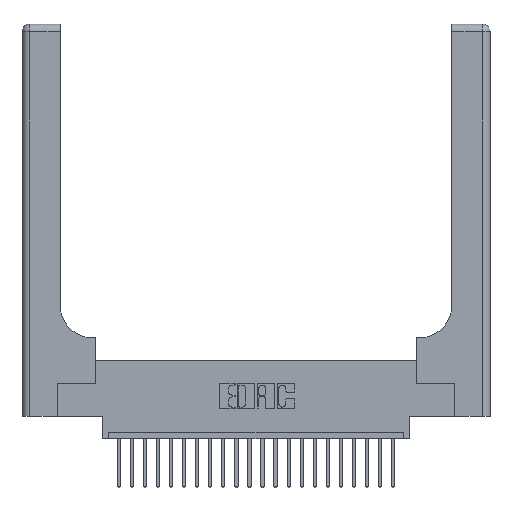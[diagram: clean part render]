
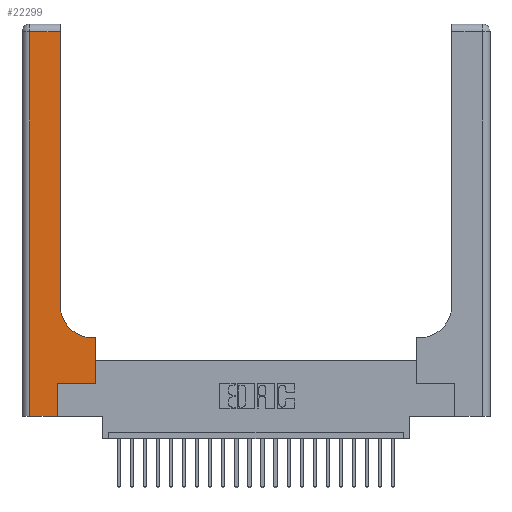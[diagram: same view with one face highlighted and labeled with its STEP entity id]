
A CAD part, top view. The second image highlights one B-rep face of the part: STEP entity #22299.
In plain terms, the highlighted planar face has unit normal (0, 0, 1).
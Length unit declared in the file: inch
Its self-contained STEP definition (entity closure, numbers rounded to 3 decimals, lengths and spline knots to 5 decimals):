
#419 = CARTESIAN_POINT ( 'NONE',  ( 0.269, 0., 0.37 ) ) ;
#493 = DIRECTION ( 'NONE',  ( 0., 0., -1. ) ) ;
#1134 = LINE ( 'NONE', #22113, #18925 ) ;
#1574 = CARTESIAN_POINT ( 'NONE',  ( 0.269, 0.25, 0.37 ) ) ;
#1707 = CARTESIAN_POINT ( 'NONE',  ( 0.06, 0., 0.37 ) ) ;
#3036 = EDGE_CURVE ( 'NONE', #19430, #3932, #19531, .T. ) ;
#3152 = EDGE_CURVE ( 'NONE', #24186, #20681, #1134, .T. ) ;
#3701 = VERTEX_POINT ( 'NONE', #11086 ) ;
#3727 = DIRECTION ( 'NONE',  ( 0., 0., -1. ) ) ;
#3932 = VERTEX_POINT ( 'NONE', #17463 ) ;
#4582 = LINE ( 'NONE', #4952, #14348 ) ;
#4693 = CARTESIAN_POINT ( 'NONE',  ( 0.5585, 0.25, 0.37 ) ) ;
#4952 = CARTESIAN_POINT ( 'NONE',  ( 0., 0., 0.37 ) ) ;
#5368 = DIRECTION ( 'NONE',  ( 1., 0., 0. ) ) ;
#5630 = PLANE ( 'NONE',  #20189 ) ;
#5796 = DIRECTION ( 'NONE',  ( 0., 1., 0. ) ) ;
#7305 = CARTESIAN_POINT ( 'NONE',  ( 0.5585, 0.25, 0.37 ) ) ;
#7680 = EDGE_CURVE ( 'NONE', #3701, #17671, #9521, .T. ) ;
#7905 = ORIENTED_EDGE ( 'NONE', *, *, #16802, .T. ) ;
#7967 = DIRECTION ( 'NONE',  ( 1., 0., 0. ) ) ;
#8793 = FACE_OUTER_BOUND ( 'NONE', #18716, .T. ) ;
#8909 = DIRECTION ( 'NONE',  ( 0., 1., 0. ) ) ;
#9008 = VECTOR ( 'NONE', #12059, 39.37008 ) ;
#9521 = LINE ( 'NONE', #18979, #13675 ) ;
#10297 = VECTOR ( 'NONE', #5368, 39.37008 ) ;
#10332 = CARTESIAN_POINT ( 'NONE',  ( 0.5415, 0.6, 0.37 ) ) ;
#10900 = ORIENTED_EDGE ( 'NONE', *, *, #15950, .T. ) ;
#10934 = EDGE_CURVE ( 'NONE', #22612, #18733, #11075, .T. ) ;
#11075 = LINE ( 'NONE', #20327, #13721 ) ;
#11086 = CARTESIAN_POINT ( 'NONE',  ( 0.2915, 0.85, 0.37 ) ) ;
#11249 = VECTOR ( 'NONE', #16111, 39.37008 ) ;
#12059 = DIRECTION ( 'NONE',  ( -1., 0., 0. ) ) ;
#13042 = LINE ( 'NONE', #17869, #11249 ) ;
#13675 = VECTOR ( 'NONE', #5796, 39.37008 ) ;
#13721 = VECTOR ( 'NONE', #16597, 39.37008 ) ;
#13752 = ORIENTED_EDGE ( 'NONE', *, *, #7680, .T. ) ;
#14348 = VECTOR ( 'NONE', #20052, 39.37008 ) ;
#14985 = DIRECTION ( 'NONE',  ( -1., 0., 0. ) ) ;
#15950 = EDGE_CURVE ( 'NONE', #22550, #3701, #22271, .T. ) ;
#16111 = DIRECTION ( 'NONE',  ( -1., 0., 0. ) ) ;
#16597 = DIRECTION ( 'NONE',  ( 0., -1., 0. ) ) ;
#16802 = EDGE_CURVE ( 'NONE', #3932, #22550, #13042, .T. ) ;
#17096 = CARTESIAN_POINT ( 'NONE',  ( 0., 3., 0.37 ) ) ;
#17460 = ORIENTED_EDGE ( 'NONE', *, *, #19940, .T. ) ;
#17463 = CARTESIAN_POINT ( 'NONE',  ( 0.5585, 0.6, 0.37 ) ) ;
#17553 = CARTESIAN_POINT ( 'NONE',  ( 0., 2.94, 0.37 ) ) ;
#17671 = VERTEX_POINT ( 'NONE', #22869 ) ;
#17728 = CARTESIAN_POINT ( 'NONE',  ( 0.06, 2.94, 0.37 ) ) ;
#17869 = CARTESIAN_POINT ( 'NONE',  ( 0.2915, 0.6, 0.37 ) ) ;
#17976 = DIRECTION ( 'NONE',  ( 0., 1., 0. ) ) ;
#18716 = EDGE_LOOP ( 'NONE', ( #13752, #22593, #24113, #17460, #22781, #20184, #22640, #7905, #10900 ) ) ;
#18733 = VERTEX_POINT ( 'NONE', #1707 ) ;
#18925 = VECTOR ( 'NONE', #8909, 39.37008 ) ;
#18929 = LINE ( 'NONE', #1574, #10297 ) ;
#18979 = CARTESIAN_POINT ( 'NONE',  ( 0.2915, 3., 0.37 ) ) ;
#19321 = CARTESIAN_POINT ( 'NONE',  ( 0.5415, 0.85, 0.37 ) ) ;
#19430 = VERTEX_POINT ( 'NONE', #7305 ) ;
#19531 = LINE ( 'NONE', #4693, #21917 ) ;
#19936 = CARTESIAN_POINT ( 'NONE',  ( 0.269, 0.25, 0.37 ) ) ;
#19940 = EDGE_CURVE ( 'NONE', #18733, #24186, #4582, .T. ) ;
#20052 = DIRECTION ( 'NONE',  ( 1., 0., 0. ) ) ;
#20184 = ORIENTED_EDGE ( 'NONE', *, *, #21861, .T. ) ;
#20189 = AXIS2_PLACEMENT_3D ( 'NONE', #17096, #3727, #14985 ) ;
#20327 = CARTESIAN_POINT ( 'NONE',  ( 0.06, 3., 0.37 ) ) ;
#20459 = EDGE_CURVE ( 'NONE', #17671, #22612, #21173, .T. ) ;
#20681 = VERTEX_POINT ( 'NONE', #19936 ) ;
#21173 = LINE ( 'NONE', #17553, #9008 ) ;
#21861 = EDGE_CURVE ( 'NONE', #20681, #19430, #18929, .T. ) ;
#21917 = VECTOR ( 'NONE', #17976, 39.37008 ) ;
#22113 = CARTESIAN_POINT ( 'NONE',  ( 0.269, 0., 0.37 ) ) ;
#22271 = CIRCLE ( 'NONE', #24080, 0.25 ) ;
#22299 = ADVANCED_FACE ( 'NONE', ( #8793 ), #5630, .F. ) ;
#22550 = VERTEX_POINT ( 'NONE', #10332 ) ;
#22593 = ORIENTED_EDGE ( 'NONE', *, *, #20459, .T. ) ;
#22612 = VERTEX_POINT ( 'NONE', #17728 ) ;
#22640 = ORIENTED_EDGE ( 'NONE', *, *, #3036, .T. ) ;
#22781 = ORIENTED_EDGE ( 'NONE', *, *, #3152, .T. ) ;
#22869 = CARTESIAN_POINT ( 'NONE',  ( 0.2915, 2.94, 0.37 ) ) ;
#24080 = AXIS2_PLACEMENT_3D ( 'NONE', #19321, #493, #7967 ) ;
#24113 = ORIENTED_EDGE ( 'NONE', *, *, #10934, .T. ) ;
#24186 = VERTEX_POINT ( 'NONE', #419 ) ;
